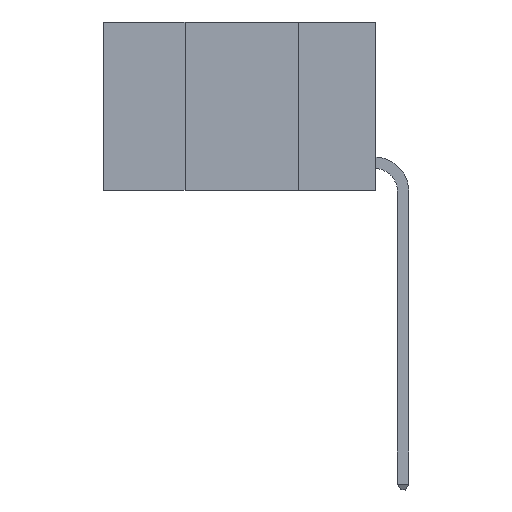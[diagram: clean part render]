
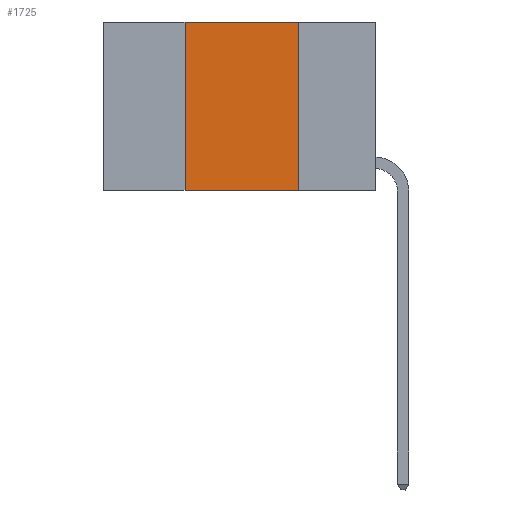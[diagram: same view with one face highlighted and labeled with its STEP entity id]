
A CAD part, left-side view. The second image highlights one B-rep face of the part: STEP entity #1725.
In plain terms, the highlighted planar face has unit normal (-1, 0, 0).
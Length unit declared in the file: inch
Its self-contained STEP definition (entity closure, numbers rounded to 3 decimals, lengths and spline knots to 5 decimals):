
#1725 = ADVANCED_FACE ( 'NONE', ( #21205 ), #17295, .F. ) ;
#1789 = AXIS2_PLACEMENT_3D ( 'NONE', #3548, #19695, #5886 ) ;
#1864 = CARTESIAN_POINT ( 'NONE',  ( 0., 0.42, 0. ) ) ;
#3411 = CARTESIAN_POINT ( 'NONE',  ( 0., 0.6, -0.37 ) ) ;
#3548 = CARTESIAN_POINT ( 'NONE',  ( 0., 0.6, 0. ) ) ;
#4224 = DIRECTION ( 'NONE',  ( 0., 0., 1. ) ) ;
#4874 = VERTEX_POINT ( 'NONE', #9166 ) ;
#5398 = ORIENTED_EDGE ( 'NONE', *, *, #27480, .F. ) ;
#5629 = LINE ( 'NONE', #1864, #23280 ) ;
#5886 = DIRECTION ( 'NONE',  ( 0., 0., -1. ) ) ;
#7584 = ORIENTED_EDGE ( 'NONE', *, *, #12166, .T. ) ;
#8322 = CARTESIAN_POINT ( 'NONE',  ( 0., 0.17, 0. ) ) ;
#9103 = CARTESIAN_POINT ( 'NONE',  ( 0., 0.42, 0. ) ) ;
#9166 = CARTESIAN_POINT ( 'NONE',  ( 0., 0.17, 0. ) ) ;
#9450 = VERTEX_POINT ( 'NONE', #9103 ) ;
#9694 = CARTESIAN_POINT ( 'NONE',  ( 0., 0.42, -0.37 ) ) ;
#10620 = DIRECTION ( 'NONE',  ( 0., 0., -1. ) ) ;
#11005 = DIRECTION ( 'NONE',  ( 0., -1., 0. ) ) ;
#12166 = EDGE_CURVE ( 'NONE', #20212, #20839, #15678, .T. ) ;
#14609 = LINE ( 'NONE', #20174, #20006 ) ;
#15352 = VECTOR ( 'NONE', #26487, 39.37008 ) ;
#15678 = LINE ( 'NONE', #3411, #15352 ) ;
#15805 = VECTOR ( 'NONE', #10620, 39.37008 ) ;
#16637 = CARTESIAN_POINT ( 'NONE',  ( 0., 0.17, -0.37 ) ) ;
#17295 = PLANE ( 'NONE',  #1789 ) ;
#17710 = EDGE_CURVE ( 'NONE', #20212, #9450, #5629, .T. ) ;
#19119 = ORIENTED_EDGE ( 'NONE', *, *, #17710, .F. ) ;
#19695 = DIRECTION ( 'NONE',  ( 1., 0., 0. ) ) ;
#20006 = VECTOR ( 'NONE', #11005, 39.37008 ) ;
#20174 = CARTESIAN_POINT ( 'NONE',  ( 0., 0.6, 0. ) ) ;
#20212 = VERTEX_POINT ( 'NONE', #9694 ) ;
#20839 = VERTEX_POINT ( 'NONE', #16637 ) ;
#21190 = LINE ( 'NONE', #8322, #15805 ) ;
#21205 = FACE_OUTER_BOUND ( 'NONE', #26974, .T. ) ;
#21875 = EDGE_CURVE ( 'NONE', #9450, #4874, #14609, .T. ) ;
#23280 = VECTOR ( 'NONE', #4224, 39.37008 ) ;
#26487 = DIRECTION ( 'NONE',  ( 0., -1., 0. ) ) ;
#26974 = EDGE_LOOP ( 'NONE', ( #5398, #29870, #19119, #7584 ) ) ;
#27480 = EDGE_CURVE ( 'NONE', #4874, #20839, #21190, .T. ) ;
#29870 = ORIENTED_EDGE ( 'NONE', *, *, #21875, .F. ) ;
